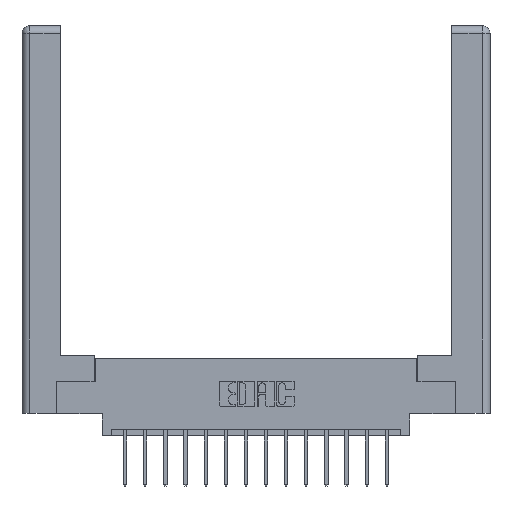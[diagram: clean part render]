
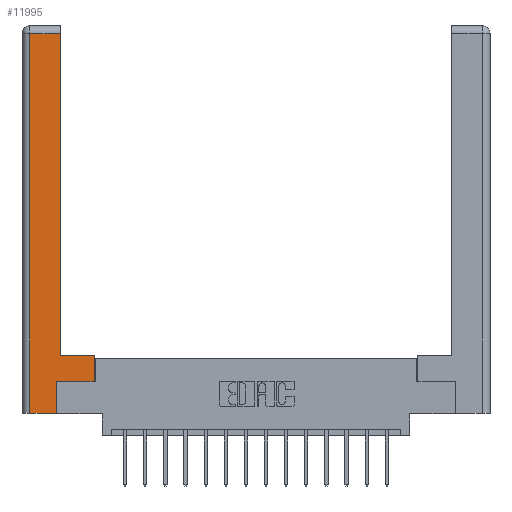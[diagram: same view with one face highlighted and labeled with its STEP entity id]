
A CAD part, top view. The second image highlights one B-rep face of the part: STEP entity #11995.
In plain terms, the highlighted planar face has unit normal (0, 0, 1).
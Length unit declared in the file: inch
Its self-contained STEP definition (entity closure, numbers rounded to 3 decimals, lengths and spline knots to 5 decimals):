
#147 = DIRECTION ( 'NONE',  ( 0., 1., 0. ) ) ;
#495 = ORIENTED_EDGE ( 'NONE', *, *, #10084, .T. ) ;
#1147 = DIRECTION ( 'NONE',  ( 0., 1., 0. ) ) ;
#1201 = CARTESIAN_POINT ( 'NONE',  ( 0.565, 0.45, 0. ) ) ;
#1575 = DIRECTION ( 'NONE',  ( 1., 0., 0. ) ) ;
#1590 = ORIENTED_EDGE ( 'NONE', *, *, #8044, .T. ) ;
#1735 = ORIENTED_EDGE ( 'NONE', *, *, #17194, .T. ) ;
#2105 = DIRECTION ( 'NONE',  ( 0., 0., -1. ) ) ;
#2258 = LINE ( 'NONE', #6508, #16856 ) ;
#2381 = CARTESIAN_POINT ( 'NONE',  ( 0.0615, 0., 0. ) ) ;
#2680 = VECTOR ( 'NONE', #3903, 39.37008 ) ;
#2920 = EDGE_CURVE ( 'NONE', #3467, #11069, #14960, .T. ) ;
#3207 = CARTESIAN_POINT ( 'NONE',  ( 0.265, 0.245, 0. ) ) ;
#3253 = LINE ( 'NONE', #1201, #5747 ) ;
#3326 = LINE ( 'NONE', #6659, #17076 ) ;
#3467 = VERTEX_POINT ( 'NONE', #5347 ) ;
#3468 = CARTESIAN_POINT ( 'NONE',  ( 0.565, 0.45, 0. ) ) ;
#3870 = CARTESIAN_POINT ( 'NONE',  ( 0.265, 0.245, 0. ) ) ;
#3903 = DIRECTION ( 'NONE',  ( -1., 0., 0. ) ) ;
#3991 = EDGE_CURVE ( 'NONE', #15437, #13077, #12817, .T. ) ;
#4237 = VECTOR ( 'NONE', #5278, 39.37008 ) ;
#4939 = EDGE_CURVE ( 'NONE', #13077, #12132, #5092, .T. ) ;
#5044 = CARTESIAN_POINT ( 'NONE',  ( 0.265, 0., 0. ) ) ;
#5092 = LINE ( 'NONE', #13266, #15318 ) ;
#5278 = DIRECTION ( 'NONE',  ( 0., -1., 0. ) ) ;
#5347 = CARTESIAN_POINT ( 'NONE',  ( 0.295, 2.94, 0. ) ) ;
#5468 = ORIENTED_EDGE ( 'NONE', *, *, #16379, .T. ) ;
#5695 = VERTEX_POINT ( 'NONE', #3468 ) ;
#5747 = VECTOR ( 'NONE', #1147, 39.37008 ) ;
#6116 = PLANE ( 'NONE',  #13242 ) ;
#6508 = CARTESIAN_POINT ( 'NONE',  ( 0.265, 0., 0. ) ) ;
#6523 = CARTESIAN_POINT ( 'NONE',  ( 0.565, 0.245, 0. ) ) ;
#6586 = VERTEX_POINT ( 'NONE', #7300 ) ;
#6659 = CARTESIAN_POINT ( 'NONE',  ( 0.295, 3., 0. ) ) ;
#6842 = DIRECTION ( 'NONE',  ( 0., 1., 0. ) ) ;
#6932 = ORIENTED_EDGE ( 'NONE', *, *, #2920, .T. ) ;
#7300 = CARTESIAN_POINT ( 'NONE',  ( 0.0615, 0., 0. ) ) ;
#7746 = EDGE_CURVE ( 'NONE', #16011, #3467, #3326, .T. ) ;
#8044 = EDGE_CURVE ( 'NONE', #6586, #15437, #2258, .T. ) ;
#8439 = VECTOR ( 'NONE', #147, 39.37008 ) ;
#8784 = FACE_OUTER_BOUND ( 'NONE', #16389, .T. ) ;
#8959 = CARTESIAN_POINT ( 'NONE',  ( 0.295, 0.45, 0. ) ) ;
#10044 = CARTESIAN_POINT ( 'NONE',  ( 0., 0., 0. ) ) ;
#10050 = VECTOR ( 'NONE', #10927, 39.37008 ) ;
#10084 = EDGE_CURVE ( 'NONE', #12132, #5695, #3253, .T. ) ;
#10213 = LINE ( 'NONE', #2381, #4237 ) ;
#10927 = DIRECTION ( 'NONE',  ( -1., 0., 0. ) ) ;
#11069 = VERTEX_POINT ( 'NONE', #16122 ) ;
#11793 = ORIENTED_EDGE ( 'NONE', *, *, #7746, .T. ) ;
#11995 = ADVANCED_FACE ( 'NONE', ( #8784 ), #6116, .F. ) ;
#12132 = VERTEX_POINT ( 'NONE', #6523 ) ;
#12745 = DIRECTION ( 'NONE',  ( -1., 0., 0. ) ) ;
#12817 = LINE ( 'NONE', #3207, #8439 ) ;
#12996 = LINE ( 'NONE', #16319, #10050 ) ;
#13025 = DIRECTION ( 'NONE',  ( 1., 0., 0. ) ) ;
#13077 = VERTEX_POINT ( 'NONE', #3870 ) ;
#13242 = AXIS2_PLACEMENT_3D ( 'NONE', #10044, #2105, #12745 ) ;
#13266 = CARTESIAN_POINT ( 'NONE',  ( 0.565, 0.245, 0. ) ) ;
#13453 = CARTESIAN_POINT ( 'NONE',  ( 0.0615, 2.94, 0. ) ) ;
#14960 = LINE ( 'NONE', #13453, #2680 ) ;
#15002 = ORIENTED_EDGE ( 'NONE', *, *, #3991, .T. ) ;
#15318 = VECTOR ( 'NONE', #1575, 39.37008 ) ;
#15437 = VERTEX_POINT ( 'NONE', #5044 ) ;
#16011 = VERTEX_POINT ( 'NONE', #8959 ) ;
#16018 = ORIENTED_EDGE ( 'NONE', *, *, #4939, .T. ) ;
#16122 = CARTESIAN_POINT ( 'NONE',  ( 0.0615, 2.94, 0. ) ) ;
#16319 = CARTESIAN_POINT ( 'NONE',  ( 0.295, 0.45, 0. ) ) ;
#16379 = EDGE_CURVE ( 'NONE', #5695, #16011, #12996, .T. ) ;
#16389 = EDGE_LOOP ( 'NONE', ( #11793, #6932, #1735, #1590, #15002, #16018, #495, #5468 ) ) ;
#16856 = VECTOR ( 'NONE', #13025, 39.37008 ) ;
#17076 = VECTOR ( 'NONE', #6842, 39.37008 ) ;
#17194 = EDGE_CURVE ( 'NONE', #11069, #6586, #10213, .T. ) ;
